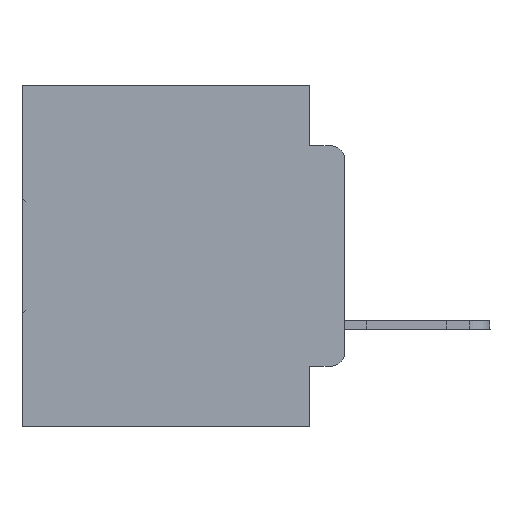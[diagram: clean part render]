
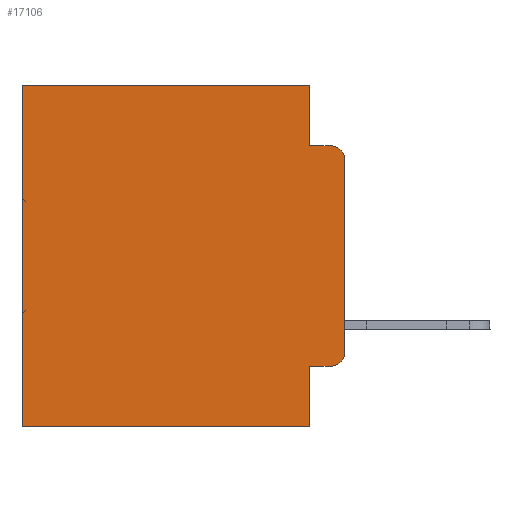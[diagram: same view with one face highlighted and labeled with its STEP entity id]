
A CAD part, left-side view. The second image highlights one B-rep face of the part: STEP entity #17106.
In plain terms, the highlighted planar face has unit normal (-1, 0, 0).
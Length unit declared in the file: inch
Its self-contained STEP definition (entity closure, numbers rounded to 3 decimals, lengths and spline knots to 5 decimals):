
#85 = LINE ( 'NONE', #20550, #4497 ) ;
#227 = ORIENTED_EDGE ( 'NONE', *, *, #1741, .F. ) ;
#267 = VECTOR ( 'NONE', #26805, 39.37008 ) ;
#678 = VERTEX_POINT ( 'NONE', #23138 ) ;
#918 = VERTEX_POINT ( 'NONE', #30166 ) ;
#1461 = ORIENTED_EDGE ( 'NONE', *, *, #3037, .T. ) ;
#1585 = DIRECTION ( 'NONE',  ( 0., 0., -1. ) ) ;
#1741 = EDGE_CURVE ( 'NONE', #11833, #918, #3576, .T. ) ;
#1765 = EDGE_LOOP ( 'NONE', ( #13444, #1461, #18471, #227, #17398, #25026, #14482, #32895, #13451, #30588 ) ) ;
#1907 = VERTEX_POINT ( 'NONE', #10615 ) ;
#2512 = CARTESIAN_POINT ( 'NONE',  ( 0.298, 0., -0.3915 ) ) ;
#2680 = VECTOR ( 'NONE', #1585, 39.37008 ) ;
#3037 = EDGE_CURVE ( 'NONE', #18046, #29917, #4728, .T. ) ;
#3067 = LINE ( 'NONE', #16009, #27411 ) ;
#3280 = CARTESIAN_POINT ( 'NONE',  ( 0.298, 0., 0. ) ) ;
#3576 = LINE ( 'NONE', #33401, #10480 ) ;
#3607 = CARTESIAN_POINT ( 'NONE',  ( 0.298, 0.02, -0.0885 ) ) ;
#4109 = VERTEX_POINT ( 'NONE', #2512 ) ;
#4497 = VECTOR ( 'NONE', #7395, 39.37008 ) ;
#4728 = CIRCLE ( 'NONE', #14844, 0.02 ) ;
#6044 = CIRCLE ( 'NONE', #16154, 0.02 ) ;
#6217 = VERTEX_POINT ( 'NONE', #16501 ) ;
#7395 = DIRECTION ( 'NONE',  ( 0., 0., -1. ) ) ;
#8653 = CARTESIAN_POINT ( 'NONE',  ( 0.298, 0.051, -0.4115 ) ) ;
#9371 = CARTESIAN_POINT ( 'NONE',  ( 0.298, 0.02, -0.1085 ) ) ;
#10480 = VECTOR ( 'NONE', #30462, 39.37008 ) ;
#10615 = CARTESIAN_POINT ( 'NONE',  ( 0.298, 0.02, -0.4115 ) ) ;
#10899 = EDGE_CURVE ( 'NONE', #18046, #4109, #10992, .T. ) ;
#10992 = LINE ( 'NONE', #3280, #26799 ) ;
#11316 = CARTESIAN_POINT ( 'NONE',  ( 0.298, 0., 0. ) ) ;
#11833 = VERTEX_POINT ( 'NONE', #18817 ) ;
#12846 = VECTOR ( 'NONE', #13482, 39.37008 ) ;
#12902 = DIRECTION ( 'NONE',  ( 1., 0., 0. ) ) ;
#13221 = LINE ( 'NONE', #8653, #267 ) ;
#13444 = ORIENTED_EDGE ( 'NONE', *, *, #10899, .F. ) ;
#13451 = ORIENTED_EDGE ( 'NONE', *, *, #21829, .T. ) ;
#13482 = DIRECTION ( 'NONE',  ( 0., 1., 0. ) ) ;
#14049 = DIRECTION ( 'NONE',  ( 0., 0., -1. ) ) ;
#14482 = ORIENTED_EDGE ( 'NONE', *, *, #22084, .F. ) ;
#14844 = AXIS2_PLACEMENT_3D ( 'NONE', #9371, #27299, #19355 ) ;
#15382 = DIRECTION ( 'NONE',  ( 0., 0., -1. ) ) ;
#16009 = CARTESIAN_POINT ( 'NONE',  ( 0.298, 0.051, -0.0885 ) ) ;
#16154 = AXIS2_PLACEMENT_3D ( 'NONE', #27962, #28075, #30698 ) ;
#16501 = CARTESIAN_POINT ( 'NONE',  ( 0.298, 0.051, -0.4115 ) ) ;
#17106 = ADVANCED_FACE ( 'NONE', ( #20750 ), #20598, .F. ) ;
#17398 = ORIENTED_EDGE ( 'NONE', *, *, #31797, .T. ) ;
#18046 = VERTEX_POINT ( 'NONE', #25598 ) ;
#18204 = CARTESIAN_POINT ( 'NONE',  ( 0.298, 0.473, -0.5 ) ) ;
#18471 = ORIENTED_EDGE ( 'NONE', *, *, #22287, .F. ) ;
#18611 = DIRECTION ( 'NONE',  ( 0., -1., 0. ) ) ;
#18817 = CARTESIAN_POINT ( 'NONE',  ( 0.298, 0.051, 0. ) ) ;
#19355 = DIRECTION ( 'NONE',  ( 0., 0., -1. ) ) ;
#20365 = CARTESIAN_POINT ( 'NONE',  ( 0.298, 0., 0. ) ) ;
#20549 = LINE ( 'NONE', #11316, #12846 ) ;
#20550 = CARTESIAN_POINT ( 'NONE',  ( 0.298, 0.473, 0. ) ) ;
#20598 = PLANE ( 'NONE',  #21080 ) ;
#20709 = EDGE_CURVE ( 'NONE', #6217, #678, #20932, .T. ) ;
#20750 = FACE_OUTER_BOUND ( 'NONE', #1765, .T. ) ;
#20932 = LINE ( 'NONE', #27546, #2680 ) ;
#21080 = AXIS2_PLACEMENT_3D ( 'NONE', #20365, #12902, #15382 ) ;
#21685 = LINE ( 'NONE', #29979, #31889 ) ;
#21829 = EDGE_CURVE ( 'NONE', #6217, #1907, #13221, .T. ) ;
#22084 = EDGE_CURVE ( 'NONE', #678, #26603, #21685, .T. ) ;
#22287 = EDGE_CURVE ( 'NONE', #918, #29917, #3067, .T. ) ;
#23138 = CARTESIAN_POINT ( 'NONE',  ( 0.298, 0.051, -0.5 ) ) ;
#24612 = CARTESIAN_POINT ( 'NONE',  ( 0.298, 0.473, 0. ) ) ;
#25026 = ORIENTED_EDGE ( 'NONE', *, *, #29028, .T. ) ;
#25598 = CARTESIAN_POINT ( 'NONE',  ( 0.298, 0., -0.1085 ) ) ;
#26603 = VERTEX_POINT ( 'NONE', #18204 ) ;
#26799 = VECTOR ( 'NONE', #14049, 39.37008 ) ;
#26805 = DIRECTION ( 'NONE',  ( 0., -1., 0. ) ) ;
#27299 = DIRECTION ( 'NONE',  ( -1., 0., 0. ) ) ;
#27411 = VECTOR ( 'NONE', #18611, 39.37008 ) ;
#27546 = CARTESIAN_POINT ( 'NONE',  ( 0.298, 0.051, 0. ) ) ;
#27962 = CARTESIAN_POINT ( 'NONE',  ( 0.298, 0.02, -0.3915 ) ) ;
#28075 = DIRECTION ( 'NONE',  ( -1., 0., 0. ) ) ;
#28366 = DIRECTION ( 'NONE',  ( 0., 1., 0. ) ) ;
#29028 = EDGE_CURVE ( 'NONE', #31222, #26603, #85, .T. ) ;
#29917 = VERTEX_POINT ( 'NONE', #3607 ) ;
#29979 = CARTESIAN_POINT ( 'NONE',  ( 0.298, 0., -0.5 ) ) ;
#30166 = CARTESIAN_POINT ( 'NONE',  ( 0.298, 0.051, -0.0885 ) ) ;
#30217 = EDGE_CURVE ( 'NONE', #1907, #4109, #6044, .T. ) ;
#30462 = DIRECTION ( 'NONE',  ( 0., 0., -1. ) ) ;
#30588 = ORIENTED_EDGE ( 'NONE', *, *, #30217, .T. ) ;
#30698 = DIRECTION ( 'NONE',  ( 0., 0., -1. ) ) ;
#31222 = VERTEX_POINT ( 'NONE', #24612 ) ;
#31797 = EDGE_CURVE ( 'NONE', #11833, #31222, #20549, .T. ) ;
#31889 = VECTOR ( 'NONE', #28366, 39.37008 ) ;
#32895 = ORIENTED_EDGE ( 'NONE', *, *, #20709, .F. ) ;
#33401 = CARTESIAN_POINT ( 'NONE',  ( 0.298, 0.051, 0. ) ) ;
